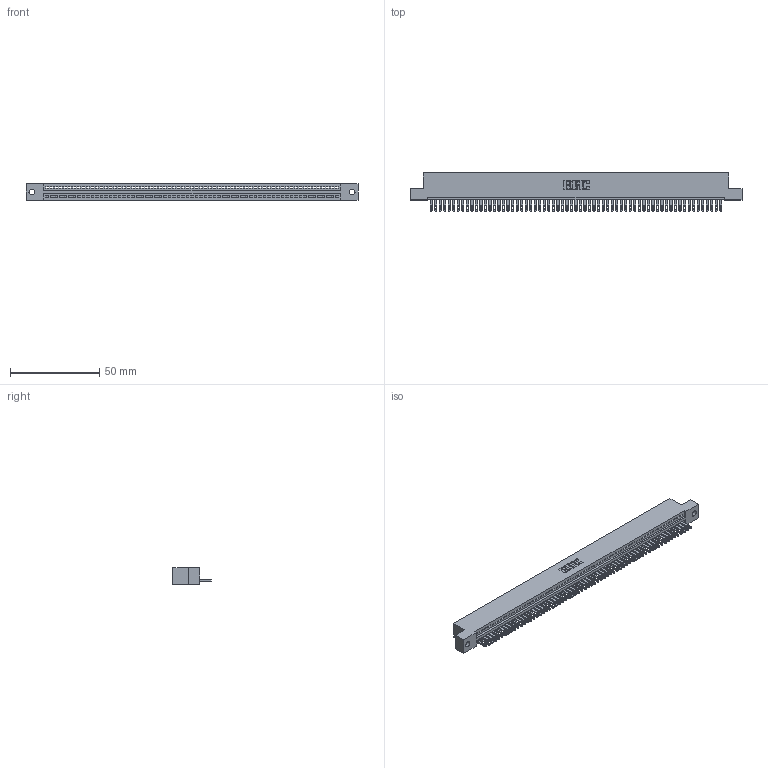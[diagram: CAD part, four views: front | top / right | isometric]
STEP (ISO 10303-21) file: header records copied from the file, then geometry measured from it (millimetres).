
FILE_DESCRIPTION (( 'STEP AP203' ), '1' );
FILE_NAME ('345-065-500-102.STEP', '2018-09-28T11:57:40', ( '' ), ( '' ), 'SwSTEP 2.0', 'SolidWorks 2016', '' );
FILE_SCHEMA (( 'CONFIG_CONTROL_DESIGN' ));
Length unit declared in the file: inch
Products named in the file (3): 345-065-500-102; 345 Part_Flush Mounting Lugs - 0.128 Dia; 345-292-001_345-293-100
Assembly tree (66 placements, depth 2):
  345-065-500-102
    345 Part_Flush Mounting Lugs - 0.128 Dia
    345-292-001_345-293-100  x65
Bounding box: 186.31 x 21.51 x 9.4 mm (x, y, z)
Volume: 17887.8 mm3; surface area: 23958.3 mm2
Topology: 66 solids, 66 shells, 3636 faces, 11261 edges, 7506 vertices
Faces by surface type: plane 2290, cylinder 1346
Entity records: 45757 total; most frequent: CARTESIAN_POINT 7931, ORIENTED_EDGE 7930, DIRECTION 6895, EDGE_CURVE 3965, LINE 3569, VECTOR 3569, VERTEX_POINT 2642, AXIS2_PLACEMENT_3D 1663
